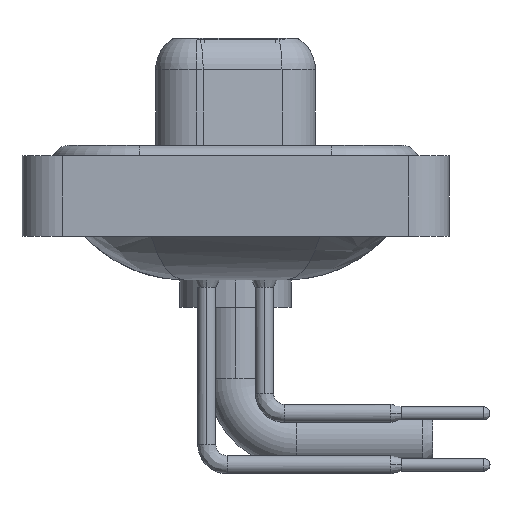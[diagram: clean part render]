
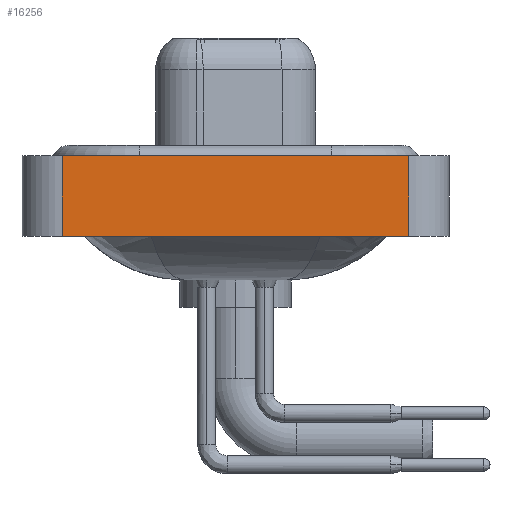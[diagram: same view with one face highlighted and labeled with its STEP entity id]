
A CAD part, left-side view. The second image highlights one B-rep face of the part: STEP entity #16256.
In plain terms, the highlighted planar face has unit normal (-1, 0, 0).
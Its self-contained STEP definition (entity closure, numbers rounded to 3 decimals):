
#123 = ORIENTED_EDGE ( 'NONE', *, *, #25444, .T. ) ;
#388 = EDGE_LOOP ( 'NONE', ( #22847, #3990, #9294, #123 ) ) ;
#994 = LINE ( 'NONE', #7509, #8808 ) ;
#1258 = DIRECTION ( 'NONE',  ( 0., -1., 0. ) ) ;
#1615 = LINE ( 'NONE', #17890, #18715 ) ;
#2606 = VERTEX_POINT ( 'NONE', #22200 ) ;
#3722 = AXIS2_PLACEMENT_3D ( 'NONE', #6529, #16421, #14683 ) ;
#3990 = ORIENTED_EDGE ( 'NONE', *, *, #17580, .F. ) ;
#6529 = CARTESIAN_POINT ( 'NONE',  ( -7.35, -8.55, -3.6 ) ) ;
#7509 = CARTESIAN_POINT ( 'NONE',  ( -7.35, -8.55, -3.6 ) ) ;
#8687 = CARTESIAN_POINT ( 'NONE',  ( -7.35, -8.55, -3.6 ) ) ;
#8808 = VECTOR ( 'NONE', #1258, 1000. ) ;
#9294 = ORIENTED_EDGE ( 'NONE', *, *, #14717, .F. ) ;
#11179 = EDGE_CURVE ( 'NONE', #2606, #12656, #24564, .T. ) ;
#11651 = CARTESIAN_POINT ( 'NONE',  ( -7.35, 8.55, -3.6 ) ) ;
#12656 = VERTEX_POINT ( 'NONE', #25092 ) ;
#13008 = CARTESIAN_POINT ( 'NONE',  ( -7.35, 8.55, 0.4 ) ) ;
#13089 = CARTESIAN_POINT ( 'NONE',  ( -7.35, -8.55, 0.4 ) ) ;
#14683 = DIRECTION ( 'NONE',  ( 0., 0., 1. ) ) ;
#14717 = EDGE_CURVE ( 'NONE', #15946, #25415, #1615, .T. ) ;
#15946 = VERTEX_POINT ( 'NONE', #11651 ) ;
#16256 = ADVANCED_FACE ( 'NONE', ( #18684 ), #24811, .T. ) ;
#16421 = DIRECTION ( 'NONE',  ( -1., 0., 0. ) ) ;
#16438 = DIRECTION ( 'NONE',  ( 0., 0., 1. ) ) ;
#17580 = EDGE_CURVE ( 'NONE', #25415, #12656, #19483, .T. ) ;
#17750 = DIRECTION ( 'NONE',  ( 0., 0., 1. ) ) ;
#17890 = CARTESIAN_POINT ( 'NONE',  ( -7.35, 8.55, -3.6 ) ) ;
#18684 = FACE_OUTER_BOUND ( 'NONE', #388, .T. ) ;
#18715 = VECTOR ( 'NONE', #17750, 1000. ) ;
#19483 = LINE ( 'NONE', #13089, #21299 ) ;
#21299 = VECTOR ( 'NONE', #21349, 1000. ) ;
#21349 = DIRECTION ( 'NONE',  ( 0., -1., 0. ) ) ;
#22200 = CARTESIAN_POINT ( 'NONE',  ( -7.35, -8.55, -3.6 ) ) ;
#22847 = ORIENTED_EDGE ( 'NONE', *, *, #11179, .T. ) ;
#24505 = VECTOR ( 'NONE', #16438, 1000. ) ;
#24564 = LINE ( 'NONE', #8687, #24505 ) ;
#24811 = PLANE ( 'NONE',  #3722 ) ;
#25092 = CARTESIAN_POINT ( 'NONE',  ( -7.35, -8.55, 0.4 ) ) ;
#25415 = VERTEX_POINT ( 'NONE', #13008 ) ;
#25444 = EDGE_CURVE ( 'NONE', #15946, #2606, #994, .T. ) ;
